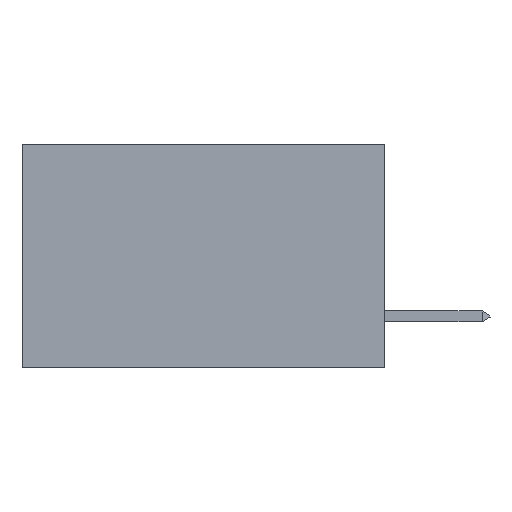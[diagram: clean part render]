
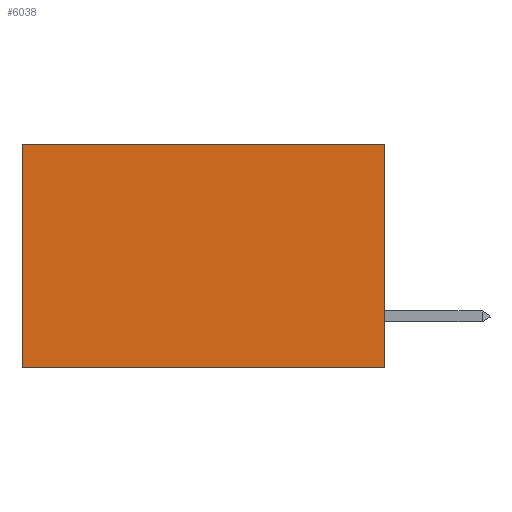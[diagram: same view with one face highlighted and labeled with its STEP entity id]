
A CAD part, left-side view. The second image highlights one B-rep face of the part: STEP entity #6038.
In plain terms, the highlighted planar face has unit normal (-1, 0, 0).
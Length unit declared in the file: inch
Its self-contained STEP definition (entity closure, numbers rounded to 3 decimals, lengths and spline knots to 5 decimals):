
#1146 = DIRECTION ( 'NONE',  ( 0., 0., -1. ) ) ;
#2117 = VERTEX_POINT ( 'NONE', #9749 ) ;
#3790 = CARTESIAN_POINT ( 'NONE',  ( 0.2875, 0.6, -0.37 ) ) ;
#4361 = VERTEX_POINT ( 'NONE', #19810 ) ;
#4484 = DIRECTION ( 'NONE',  ( 0., 0., -1. ) ) ;
#6038 = ADVANCED_FACE ( 'NONE', ( #25279 ), #25426, .F. ) ;
#6927 = CARTESIAN_POINT ( 'NONE',  ( 0.2875, 0.6, 0. ) ) ;
#7927 = DIRECTION ( 'NONE',  ( 0., 1., 0. ) ) ;
#8292 = VECTOR ( 'NONE', #26092, 39.37008 ) ;
#8716 = ORIENTED_EDGE ( 'NONE', *, *, #21837, .T. ) ;
#8898 = VERTEX_POINT ( 'NONE', #10794 ) ;
#9749 = CARTESIAN_POINT ( 'NONE',  ( 0.2875, 0.6, 0. ) ) ;
#10015 = EDGE_CURVE ( 'NONE', #4361, #8898, #16794, .T. ) ;
#10794 = CARTESIAN_POINT ( 'NONE',  ( 0.2875, 0., -0.37 ) ) ;
#11000 = ORIENTED_EDGE ( 'NONE', *, *, #10015, .F. ) ;
#11112 = EDGE_LOOP ( 'NONE', ( #15506, #26141, #11000, #8716 ) ) ;
#12519 = LINE ( 'NONE', #6927, #30231 ) ;
#12814 = EDGE_CURVE ( 'NONE', #8898, #30299, #17507, .T. ) ;
#15506 = ORIENTED_EDGE ( 'NONE', *, *, #29210, .T. ) ;
#15870 = DIRECTION ( 'NONE',  ( 1., 0., 0. ) ) ;
#16794 = LINE ( 'NONE', #19819, #22439 ) ;
#17507 = LINE ( 'NONE', #22531, #25385 ) ;
#19810 = CARTESIAN_POINT ( 'NONE',  ( 0.2875, 0., 0. ) ) ;
#19819 = CARTESIAN_POINT ( 'NONE',  ( 0.2875, 0., 0. ) ) ;
#21837 = EDGE_CURVE ( 'NONE', #4361, #2117, #27627, .T. ) ;
#21865 = AXIS2_PLACEMENT_3D ( 'NONE', #23028, #15870, #1146 ) ;
#22439 = VECTOR ( 'NONE', #29533, 39.37008 ) ;
#22531 = CARTESIAN_POINT ( 'NONE',  ( 0.2875, 0., -0.37 ) ) ;
#23028 = CARTESIAN_POINT ( 'NONE',  ( 0.2875, 0., 0. ) ) ;
#23673 = CARTESIAN_POINT ( 'NONE',  ( 0.2875, 0., 0. ) ) ;
#25279 = FACE_OUTER_BOUND ( 'NONE', #11112, .T. ) ;
#25385 = VECTOR ( 'NONE', #7927, 39.37008 ) ;
#25426 = PLANE ( 'NONE',  #21865 ) ;
#26092 = DIRECTION ( 'NONE',  ( 0., 1., 0. ) ) ;
#26141 = ORIENTED_EDGE ( 'NONE', *, *, #12814, .F. ) ;
#27627 = LINE ( 'NONE', #23673, #8292 ) ;
#29210 = EDGE_CURVE ( 'NONE', #2117, #30299, #12519, .T. ) ;
#29533 = DIRECTION ( 'NONE',  ( 0., 0., -1. ) ) ;
#30231 = VECTOR ( 'NONE', #4484, 39.37008 ) ;
#30299 = VERTEX_POINT ( 'NONE', #3790 ) ;
